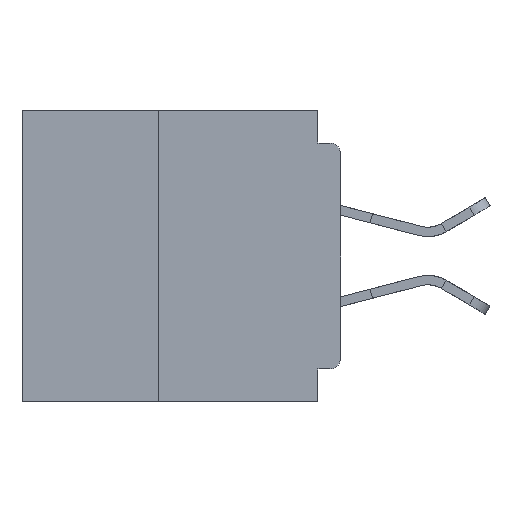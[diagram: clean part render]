
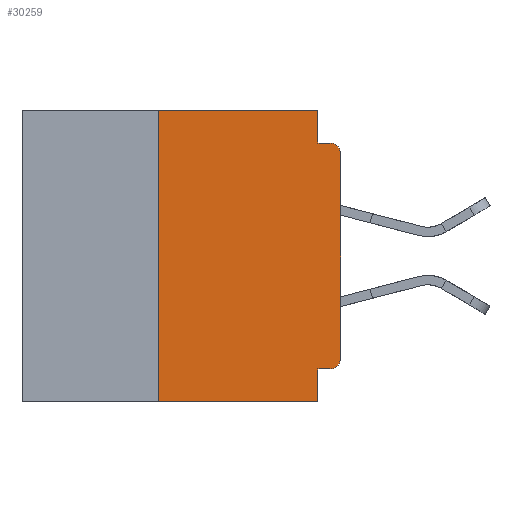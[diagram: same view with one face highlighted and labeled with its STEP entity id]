
A CAD part, left-side view. The second image highlights one B-rep face of the part: STEP entity #30259.
In plain terms, the highlighted planar face has unit normal (-1, 0, 0).
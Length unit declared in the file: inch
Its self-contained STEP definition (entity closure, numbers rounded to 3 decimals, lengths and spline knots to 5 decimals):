
#456 = VERTEX_POINT ( 'NONE', #8677 ) ;
#563 = DIRECTION ( 'NONE',  ( 1., 0., 0. ) ) ;
#829 = LINE ( 'NONE', #14608, #24483 ) ;
#870 = EDGE_CURVE ( 'NONE', #26087, #31422, #13944, .T. ) ;
#946 = CARTESIAN_POINT ( 'NONE',  ( 0., 0.031, -0.4 ) ) ;
#1778 = VECTOR ( 'NONE', #20985, 39.37008 ) ;
#2500 = CARTESIAN_POINT ( 'NONE',  ( 0., 0., -0.045 ) ) ;
#2601 = ORIENTED_EDGE ( 'NONE', *, *, #870, .T. ) ;
#3426 = CARTESIAN_POINT ( 'NONE',  ( 0., 0.031, -0.045 ) ) ;
#3751 = VECTOR ( 'NONE', #39047, 39.37008 ) ;
#4996 = DIRECTION ( 'NONE',  ( -1., 0., 0. ) ) ;
#5282 = ORIENTED_EDGE ( 'NONE', *, *, #35323, .T. ) ;
#5295 = DIRECTION ( 'NONE',  ( 0., 1., 0. ) ) ;
#5886 = CARTESIAN_POINT ( 'NONE',  ( 0., 0.437, 0. ) ) ;
#6430 = DIRECTION ( 'NONE',  ( 0., 0., 1. ) ) ;
#6738 = CARTESIAN_POINT ( 'NONE',  ( 0., 0.015, -0.355 ) ) ;
#6980 = VERTEX_POINT ( 'NONE', #28257 ) ;
#7106 = DIRECTION ( 'NONE',  ( 0., 0., -1. ) ) ;
#7191 = FACE_OUTER_BOUND ( 'NONE', #35758, .T. ) ;
#7370 = VERTEX_POINT ( 'NONE', #39303 ) ;
#8677 = CARTESIAN_POINT ( 'NONE',  ( 0., 0.031, -0.4 ) ) ;
#8993 = DIRECTION ( 'NONE',  ( 0., -1., 0. ) ) ;
#9163 = CARTESIAN_POINT ( 'NONE',  ( 0., 0.031, 0. ) ) ;
#10181 = DIRECTION ( 'NONE',  ( -1., 0., 0. ) ) ;
#10458 = VECTOR ( 'NONE', #13761, 39.37008 ) ;
#10808 = CARTESIAN_POINT ( 'NONE',  ( 0., 0., 0. ) ) ;
#10953 = CARTESIAN_POINT ( 'NONE',  ( 0., 0.031, -0.355 ) ) ;
#11538 = LINE ( 'NONE', #946, #19695 ) ;
#12085 = ORIENTED_EDGE ( 'NONE', *, *, #31736, .T. ) ;
#12675 = VECTOR ( 'NONE', #24507, 39.37008 ) ;
#13600 = VERTEX_POINT ( 'NONE', #6738 ) ;
#13761 = DIRECTION ( 'NONE',  ( 0., -1., 0. ) ) ;
#13801 = CARTESIAN_POINT ( 'NONE',  ( 0., 0., -0.34 ) ) ;
#13944 = LINE ( 'NONE', #10808, #3751 ) ;
#14608 = CARTESIAN_POINT ( 'NONE',  ( 0., 0., -0.355 ) ) ;
#14611 = ORIENTED_EDGE ( 'NONE', *, *, #30624, .F. ) ;
#15404 = CARTESIAN_POINT ( 'NONE',  ( 0., 0.031, 0. ) ) ;
#15998 = EDGE_CURVE ( 'NONE', #13600, #26087, #24800, .T. ) ;
#16029 = PLANE ( 'NONE',  #19099 ) ;
#16520 = EDGE_CURVE ( 'NONE', #6980, #25339, #28129, .T. ) ;
#16734 = ORIENTED_EDGE ( 'NONE', *, *, #15998, .T. ) ;
#18228 = ORIENTED_EDGE ( 'NONE', *, *, #16520, .F. ) ;
#19099 = AXIS2_PLACEMENT_3D ( 'NONE', #22077, #563, #22207 ) ;
#19209 = LINE ( 'NONE', #2500, #1778 ) ;
#19695 = VECTOR ( 'NONE', #7106, 39.37008 ) ;
#19799 = EDGE_CURVE ( 'NONE', #25339, #33392, #32175, .T. ) ;
#20985 = DIRECTION ( 'NONE',  ( 0., -1., 0. ) ) ;
#21298 = ORIENTED_EDGE ( 'NONE', *, *, #34946, .F. ) ;
#21778 = LINE ( 'NONE', #15404, #12675 ) ;
#21903 = VECTOR ( 'NONE', #6430, 39.37008 ) ;
#22077 = CARTESIAN_POINT ( 'NONE',  ( 0., 0.437, 0. ) ) ;
#22207 = DIRECTION ( 'NONE',  ( 0., 0., -1. ) ) ;
#22567 = ORIENTED_EDGE ( 'NONE', *, *, #19799, .F. ) ;
#22819 = EDGE_CURVE ( 'NONE', #26099, #456, #11538, .T. ) ;
#23395 = CARTESIAN_POINT ( 'NONE',  ( 0., 0.015, -0.06 ) ) ;
#24483 = VECTOR ( 'NONE', #5295, 39.37008 ) ;
#24507 = DIRECTION ( 'NONE',  ( 0., 0., -1. ) ) ;
#24800 = CIRCLE ( 'NONE', #35603, 0.015 ) ;
#24806 = CARTESIAN_POINT ( 'NONE',  ( 0., 0.25, -0.4 ) ) ;
#25339 = VERTEX_POINT ( 'NONE', #34437 ) ;
#26087 = VERTEX_POINT ( 'NONE', #13801 ) ;
#26099 = VERTEX_POINT ( 'NONE', #10953 ) ;
#26161 = ORIENTED_EDGE ( 'NONE', *, *, #22819, .F. ) ;
#26504 = DIRECTION ( 'NONE',  ( 0., 0., -1. ) ) ;
#26762 = LINE ( 'NONE', #32097, #10458 ) ;
#27562 = CARTESIAN_POINT ( 'NONE',  ( 0., 0., -0.06 ) ) ;
#28129 = LINE ( 'NONE', #24806, #21903 ) ;
#28257 = CARTESIAN_POINT ( 'NONE',  ( 0., 0.25, -0.4 ) ) ;
#28561 = CARTESIAN_POINT ( 'NONE',  ( 0., 0.015, -0.34 ) ) ;
#30259 = ADVANCED_FACE ( 'NONE', ( #7191 ), #16029, .F. ) ;
#30624 = EDGE_CURVE ( 'NONE', #30797, #7370, #19209, .T. ) ;
#30797 = VERTEX_POINT ( 'NONE', #3426 ) ;
#30841 = CIRCLE ( 'NONE', #37680, 0.015 ) ;
#31422 = VERTEX_POINT ( 'NONE', #27562 ) ;
#31622 = DIRECTION ( 'NONE',  ( 0., 0., -1. ) ) ;
#31736 = EDGE_CURVE ( 'NONE', #6980, #456, #26762, .T. ) ;
#32097 = CARTESIAN_POINT ( 'NONE',  ( 0., 0.437, -0.4 ) ) ;
#32175 = LINE ( 'NONE', #5886, #39326 ) ;
#33101 = ORIENTED_EDGE ( 'NONE', *, *, #37269, .F. ) ;
#33392 = VERTEX_POINT ( 'NONE', #9163 ) ;
#34437 = CARTESIAN_POINT ( 'NONE',  ( 0., 0.25, 0. ) ) ;
#34946 = EDGE_CURVE ( 'NONE', #33392, #30797, #21778, .T. ) ;
#35323 = EDGE_CURVE ( 'NONE', #31422, #7370, #30841, .T. ) ;
#35603 = AXIS2_PLACEMENT_3D ( 'NONE', #28561, #10181, #31622 ) ;
#35758 = EDGE_LOOP ( 'NONE', ( #2601, #5282, #14611, #21298, #22567, #18228, #12085, #26161, #33101, #16734 ) ) ;
#37269 = EDGE_CURVE ( 'NONE', #13600, #26099, #829, .T. ) ;
#37680 = AXIS2_PLACEMENT_3D ( 'NONE', #23395, #4996, #26504 ) ;
#39047 = DIRECTION ( 'NONE',  ( 0., 0., 1. ) ) ;
#39303 = CARTESIAN_POINT ( 'NONE',  ( 0., 0.015, -0.045 ) ) ;
#39326 = VECTOR ( 'NONE', #8993, 39.37008 ) ;
